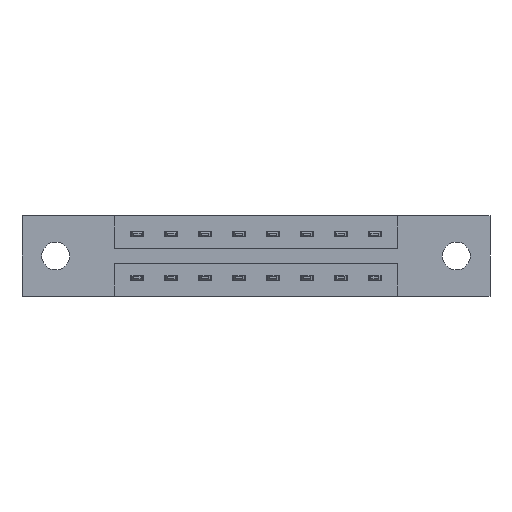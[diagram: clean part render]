
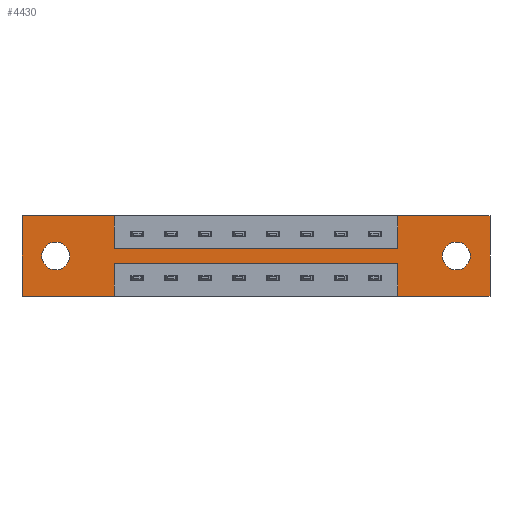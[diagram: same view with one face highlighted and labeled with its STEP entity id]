
A CAD part, front view. The second image highlights one B-rep face of the part: STEP entity #4430.
In plain terms, the highlighted planar face has unit normal (0, -1, 0).
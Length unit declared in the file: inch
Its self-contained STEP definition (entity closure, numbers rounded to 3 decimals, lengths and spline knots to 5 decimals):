
#86 = DIRECTION ( 'NONE',  ( 0., 0., -1. ) ) ;
#137 = CARTESIAN_POINT ( 'NONE',  ( 1.729, 0., -0.15 ) ) ;
#487 = CARTESIAN_POINT ( 'NONE',  ( 0.155, 0., -0.185 ) ) ;
#720 = VERTEX_POINT ( 'NONE', #7710 ) ;
#745 = EDGE_CURVE ( 'NONE', #8796, #6717, #6335, .T. ) ;
#788 = EDGE_CURVE ( 'NONE', #9134, #4199, #5819, .T. ) ;
#861 = CARTESIAN_POINT ( 'NONE',  ( 0., 0., -0.37 ) ) ;
#985 = VERTEX_POINT ( 'NONE', #3514 ) ;
#1008 = VERTEX_POINT ( 'NONE', #8906 ) ;
#1087 = VERTEX_POINT ( 'NONE', #1105 ) ;
#1105 = CARTESIAN_POINT ( 'NONE',  ( 1.999, 0., -0.249 ) ) ;
#1361 = ORIENTED_EDGE ( 'NONE', *, *, #2067, .F. ) ;
#1442 = LINE ( 'NONE', #4997, #7286 ) ;
#1470 = DIRECTION ( 'NONE',  ( 1., 0., 0. ) ) ;
#1519 = DIRECTION ( 'NONE',  ( 0., 1., 0. ) ) ;
#1717 = CARTESIAN_POINT ( 'NONE',  ( 0.425, 0., -0.22 ) ) ;
#1804 = CARTESIAN_POINT ( 'NONE',  ( 0.425, 0., -0.22 ) ) ;
#1842 = DIRECTION ( 'NONE',  ( 0., 0., 1. ) ) ;
#1863 = ORIENTED_EDGE ( 'NONE', *, *, #3782, .T. ) ;
#1879 = DIRECTION ( 'NONE',  ( 0., 0., 1. ) ) ;
#1943 = VECTOR ( 'NONE', #1470, 39.37008 ) ;
#2007 = ORIENTED_EDGE ( 'NONE', *, *, #4817, .T. ) ;
#2067 = EDGE_CURVE ( 'NONE', #720, #8796, #6185, .T. ) ;
#2413 = AXIS2_PLACEMENT_3D ( 'NONE', #3679, #7649, #9345 ) ;
#2429 = CARTESIAN_POINT ( 'NONE',  ( 0., 0., 0. ) ) ;
#2541 = CARTESIAN_POINT ( 'NONE',  ( 1.999, 0., -0.185 ) ) ;
#2545 = VERTEX_POINT ( 'NONE', #6394 ) ;
#2634 = EDGE_CURVE ( 'NONE', #6717, #8647, #1442, .T. ) ;
#2728 = CARTESIAN_POINT ( 'NONE',  ( 1.729, 0., -0.22 ) ) ;
#2752 = CARTESIAN_POINT ( 'NONE',  ( 1.729, 0., -0.37 ) ) ;
#2854 = AXIS2_PLACEMENT_3D ( 'NONE', #6318, #1519, #7097 ) ;
#2869 = CARTESIAN_POINT ( 'NONE',  ( 0.425, 0., -0.15 ) ) ;
#2941 = CARTESIAN_POINT ( 'NONE',  ( 0.425, 0., -0.15 ) ) ;
#3164 = CARTESIAN_POINT ( 'NONE',  ( 0.425, 0., -0.37 ) ) ;
#3200 = VERTEX_POINT ( 'NONE', #3203 ) ;
#3203 = CARTESIAN_POINT ( 'NONE',  ( 1.729, 0., -0.37 ) ) ;
#3252 = CARTESIAN_POINT ( 'NONE',  ( 2.154, 0., -0.37 ) ) ;
#3254 = CARTESIAN_POINT ( 'NONE',  ( 0., 0., 0. ) ) ;
#3282 = CIRCLE ( 'NONE', #4631, 0.064 ) ;
#3344 = VERTEX_POINT ( 'NONE', #4451 ) ;
#3514 = CARTESIAN_POINT ( 'NONE',  ( 0.155, 0., -0.249 ) ) ;
#3541 = VECTOR ( 'NONE', #4752, 39.37008 ) ;
#3679 = CARTESIAN_POINT ( 'NONE',  ( 0., 0., -0.37 ) ) ;
#3719 = ORIENTED_EDGE ( 'NONE', *, *, #5880, .F. ) ;
#3753 = DIRECTION ( 'NONE',  ( 0., 0., 1. ) ) ;
#3782 = EDGE_CURVE ( 'NONE', #1008, #985, #6783, .T. ) ;
#3784 = VECTOR ( 'NONE', #8940, 39.37008 ) ;
#3801 = CARTESIAN_POINT ( 'NONE',  ( 0.425, 0., 0. ) ) ;
#3824 = VECTOR ( 'NONE', #9731, 39.37008 ) ;
#3887 = CARTESIAN_POINT ( 'NONE',  ( 1.999, 0., -0.121 ) ) ;
#3919 = EDGE_CURVE ( 'NONE', #4489, #3344, #9434, .T. ) ;
#4199 = VERTEX_POINT ( 'NONE', #3164 ) ;
#4212 = EDGE_LOOP ( 'NONE', ( #1863, #7636 ) ) ;
#4261 = DIRECTION ( 'NONE',  ( -1., 0., 0. ) ) ;
#4317 = EDGE_LOOP ( 'NONE', ( #5110, #2007 ) ) ;
#4366 = VERTEX_POINT ( 'NONE', #2728 ) ;
#4419 = EDGE_LOOP ( 'NONE', ( #8644, #7932, #7686, #4491, #9153, #9308, #4604, #6409, #1361, #5455, #4562, #3719 ) ) ;
#4430 = ADVANCED_FACE ( 'NONE', ( #6902, #4989, #7258 ), #6113, .T. ) ;
#4451 = CARTESIAN_POINT ( 'NONE',  ( 0., 0., 0. ) ) ;
#4460 = LINE ( 'NONE', #7326, #5056 ) ;
#4489 = VERTEX_POINT ( 'NONE', #8407 ) ;
#4491 = ORIENTED_EDGE ( 'NONE', *, *, #4569, .F. ) ;
#4562 = ORIENTED_EDGE ( 'NONE', *, *, #3919, .F. ) ;
#4569 = EDGE_CURVE ( 'NONE', #4845, #3200, #6644, .T. ) ;
#4604 = ORIENTED_EDGE ( 'NONE', *, *, #2634, .F. ) ;
#4618 = VECTOR ( 'NONE', #1879, 39.37008 ) ;
#4631 = AXIS2_PLACEMENT_3D ( 'NONE', #487, #10140, #3753 ) ;
#4752 = DIRECTION ( 'NONE',  ( 0., 0., -1. ) ) ;
#4817 = EDGE_CURVE ( 'NONE', #1087, #6566, #8913, .T. ) ;
#4845 = VERTEX_POINT ( 'NONE', #3252 ) ;
#4887 = VECTOR ( 'NONE', #9469, 39.37008 ) ;
#4989 = FACE_BOUND ( 'NONE', #4212, .T. ) ;
#4997 = CARTESIAN_POINT ( 'NONE',  ( 1.729, 0., 0. ) ) ;
#5049 = VECTOR ( 'NONE', #9186, 39.37008 ) ;
#5056 = VECTOR ( 'NONE', #8220, 39.37008 ) ;
#5110 = ORIENTED_EDGE ( 'NONE', *, *, #7242, .T. ) ;
#5216 = DIRECTION ( 'NONE',  ( -1., 0., 0. ) ) ;
#5455 = ORIENTED_EDGE ( 'NONE', *, *, #6768, .F. ) ;
#5496 = EDGE_CURVE ( 'NONE', #8647, #2545, #10052, .T. ) ;
#5742 = VECTOR ( 'NONE', #7976, 39.37008 ) ;
#5819 = LINE ( 'NONE', #7136, #3541 ) ;
#5880 = EDGE_CURVE ( 'NONE', #4199, #4489, #7341, .T. ) ;
#5981 = CIRCLE ( 'NONE', #9088, 0.064 ) ;
#6039 = CARTESIAN_POINT ( 'NONE',  ( 0., 0., -0.37 ) ) ;
#6113 = PLANE ( 'NONE',  #2413 ) ;
#6185 = LINE ( 'NONE', #3801, #4887 ) ;
#6318 = CARTESIAN_POINT ( 'NONE',  ( 0.155, 0., -0.185 ) ) ;
#6329 = VECTOR ( 'NONE', #4261, 39.37008 ) ;
#6335 = LINE ( 'NONE', #2941, #1943 ) ;
#6370 = CARTESIAN_POINT ( 'NONE',  ( 1.729, 0., 0. ) ) ;
#6394 = CARTESIAN_POINT ( 'NONE',  ( 2.154, 0., 0. ) ) ;
#6409 = ORIENTED_EDGE ( 'NONE', *, *, #745, .F. ) ;
#6566 = VERTEX_POINT ( 'NONE', #3887 ) ;
#6630 = CARTESIAN_POINT ( 'NONE',  ( 1.999, 0., -0.185 ) ) ;
#6644 = LINE ( 'NONE', #6039, #9781 ) ;
#6693 = LINE ( 'NONE', #7967, #3784 ) ;
#6717 = VERTEX_POINT ( 'NONE', #137 ) ;
#6768 = EDGE_CURVE ( 'NONE', #3344, #720, #4460, .T. ) ;
#6783 = CIRCLE ( 'NONE', #2854, 0.064 ) ;
#6902 = FACE_BOUND ( 'NONE', #4317, .T. ) ;
#7097 = DIRECTION ( 'NONE',  ( 0., 0., 1. ) ) ;
#7136 = CARTESIAN_POINT ( 'NONE',  ( 0.425, 0., -0.37 ) ) ;
#7242 = EDGE_CURVE ( 'NONE', #6566, #1087, #5981, .T. ) ;
#7258 = FACE_OUTER_BOUND ( 'NONE', #4419, .T. ) ;
#7286 = VECTOR ( 'NONE', #1842, 39.37008 ) ;
#7326 = CARTESIAN_POINT ( 'NONE',  ( 0., 0., 0. ) ) ;
#7341 = LINE ( 'NONE', #861, #3824 ) ;
#7363 = EDGE_CURVE ( 'NONE', #3200, #4366, #9236, .T. ) ;
#7636 = ORIENTED_EDGE ( 'NONE', *, *, #8980, .T. ) ;
#7649 = DIRECTION ( 'NONE',  ( 0., -1., 0. ) ) ;
#7686 = ORIENTED_EDGE ( 'NONE', *, *, #7363, .F. ) ;
#7710 = CARTESIAN_POINT ( 'NONE',  ( 0.425, 0., 0. ) ) ;
#7931 = LINE ( 'NONE', #1804, #6329 ) ;
#7932 = ORIENTED_EDGE ( 'NONE', *, *, #8126, .F. ) ;
#7967 = CARTESIAN_POINT ( 'NONE',  ( 2.154, 0., 0. ) ) ;
#7976 = DIRECTION ( 'NONE',  ( 1., 0., 0. ) ) ;
#8102 = DIRECTION ( 'NONE',  ( 0., 1., 0. ) ) ;
#8126 = EDGE_CURVE ( 'NONE', #4366, #9134, #7931, .T. ) ;
#8220 = DIRECTION ( 'NONE',  ( 1., 0., 0. ) ) ;
#8407 = CARTESIAN_POINT ( 'NONE',  ( 0., 0., -0.37 ) ) ;
#8644 = ORIENTED_EDGE ( 'NONE', *, *, #788, .F. ) ;
#8647 = VERTEX_POINT ( 'NONE', #6370 ) ;
#8796 = VERTEX_POINT ( 'NONE', #2869 ) ;
#8894 = DIRECTION ( 'NONE',  ( 0., 1., 0. ) ) ;
#8906 = CARTESIAN_POINT ( 'NONE',  ( 0.155, 0., -0.121 ) ) ;
#8913 = CIRCLE ( 'NONE', #9962, 0.064 ) ;
#8935 = DIRECTION ( 'NONE',  ( 0., 0., -1. ) ) ;
#8940 = DIRECTION ( 'NONE',  ( 0., 0., -1. ) ) ;
#8980 = EDGE_CURVE ( 'NONE', #985, #1008, #3282, .T. ) ;
#9088 = AXIS2_PLACEMENT_3D ( 'NONE', #6630, #8894, #86 ) ;
#9134 = VERTEX_POINT ( 'NONE', #1717 ) ;
#9153 = ORIENTED_EDGE ( 'NONE', *, *, #9184, .F. ) ;
#9184 = EDGE_CURVE ( 'NONE', #2545, #4845, #6693, .T. ) ;
#9186 = DIRECTION ( 'NONE',  ( 0., 0., 1. ) ) ;
#9236 = LINE ( 'NONE', #2752, #5049 ) ;
#9308 = ORIENTED_EDGE ( 'NONE', *, *, #5496, .F. ) ;
#9345 = DIRECTION ( 'NONE',  ( 0., 0., -1. ) ) ;
#9434 = LINE ( 'NONE', #3254, #4618 ) ;
#9469 = DIRECTION ( 'NONE',  ( 0., 0., -1. ) ) ;
#9731 = DIRECTION ( 'NONE',  ( -1., 0., 0. ) ) ;
#9781 = VECTOR ( 'NONE', #5216, 39.37008 ) ;
#9962 = AXIS2_PLACEMENT_3D ( 'NONE', #2541, #8102, #8935 ) ;
#10052 = LINE ( 'NONE', #2429, #5742 ) ;
#10140 = DIRECTION ( 'NONE',  ( 0., 1., 0. ) ) ;
